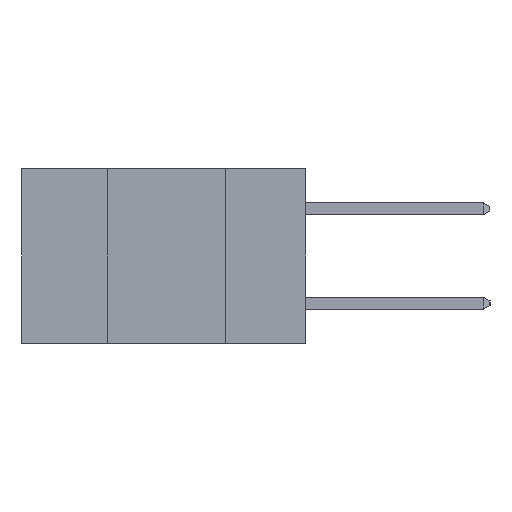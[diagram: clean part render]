
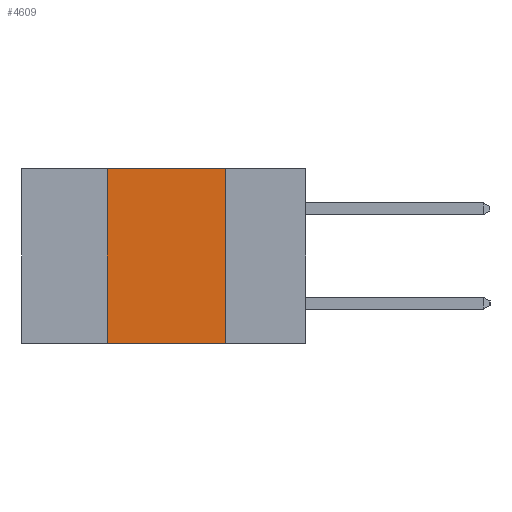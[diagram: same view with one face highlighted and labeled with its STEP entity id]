
A CAD part, left-side view. The second image highlights one B-rep face of the part: STEP entity #4609.
In plain terms, the highlighted planar face has unit normal (-1, 0, 0).
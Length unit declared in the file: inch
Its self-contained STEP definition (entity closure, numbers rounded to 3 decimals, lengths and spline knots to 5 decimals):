
#652 = DIRECTION ( 'NONE',  ( 0., -1., 0. ) ) ;
#805 = VECTOR ( 'NONE', #652, 39.37008 ) ;
#1482 = CARTESIAN_POINT ( 'NONE',  ( 0., 0.42, -0.37 ) ) ;
#1682 = VECTOR ( 'NONE', #14644, 39.37008 ) ;
#4322 = ORIENTED_EDGE ( 'NONE', *, *, #8999, .F. ) ;
#4609 = ADVANCED_FACE ( 'NONE', ( #6214 ), #9870, .F. ) ;
#5318 = LINE ( 'NONE', #13838, #805 ) ;
#5626 = EDGE_CURVE ( 'NONE', #5930, #16986, #20087, .T. ) ;
#5930 = VERTEX_POINT ( 'NONE', #12626 ) ;
#6214 = FACE_OUTER_BOUND ( 'NONE', #10781, .T. ) ;
#6602 = ORIENTED_EDGE ( 'NONE', *, *, #11107, .T. ) ;
#7385 = VECTOR ( 'NONE', #15080, 39.37008 ) ;
#7752 = ORIENTED_EDGE ( 'NONE', *, *, #5626, .F. ) ;
#8999 = EDGE_CURVE ( 'NONE', #17703, #5930, #10541, .T. ) ;
#9527 = DIRECTION ( 'NONE',  ( 1., 0., 0. ) ) ;
#9698 = DIRECTION ( 'NONE',  ( 0., 0., -1. ) ) ;
#9870 = PLANE ( 'NONE',  #14585 ) ;
#10015 = ORIENTED_EDGE ( 'NONE', *, *, #16473, .F. ) ;
#10120 = CARTESIAN_POINT ( 'NONE',  ( 0., 0.6, 0. ) ) ;
#10526 = VERTEX_POINT ( 'NONE', #15147 ) ;
#10541 = LINE ( 'NONE', #11433, #1682 ) ;
#10781 = EDGE_LOOP ( 'NONE', ( #7752, #4322, #10015, #6602 ) ) ;
#11107 = EDGE_CURVE ( 'NONE', #10526, #16986, #5318, .T. ) ;
#11400 = DIRECTION ( 'NONE',  ( 0., 0., 1. ) ) ;
#11401 = CARTESIAN_POINT ( 'NONE',  ( 0., 0.42, 0. ) ) ;
#11433 = CARTESIAN_POINT ( 'NONE',  ( 0., 0.6, 0. ) ) ;
#11652 = VECTOR ( 'NONE', #11400, 39.37008 ) ;
#12626 = CARTESIAN_POINT ( 'NONE',  ( 0., 0.17, 0. ) ) ;
#13838 = CARTESIAN_POINT ( 'NONE',  ( 0., 0.6, -0.37 ) ) ;
#14585 = AXIS2_PLACEMENT_3D ( 'NONE', #10120, #9527, #9698 ) ;
#14644 = DIRECTION ( 'NONE',  ( 0., -1., 0. ) ) ;
#15080 = DIRECTION ( 'NONE',  ( 0., 0., -1. ) ) ;
#15147 = CARTESIAN_POINT ( 'NONE',  ( 0., 0.42, -0.37 ) ) ;
#15243 = CARTESIAN_POINT ( 'NONE',  ( 0., 0.17, -0.37 ) ) ;
#15881 = LINE ( 'NONE', #1482, #11652 ) ;
#16473 = EDGE_CURVE ( 'NONE', #10526, #17703, #15881, .T. ) ;
#16986 = VERTEX_POINT ( 'NONE', #19209 ) ;
#17703 = VERTEX_POINT ( 'NONE', #11401 ) ;
#19209 = CARTESIAN_POINT ( 'NONE',  ( 0., 0.17, -0.37 ) ) ;
#20087 = LINE ( 'NONE', #15243, #7385 ) ;
